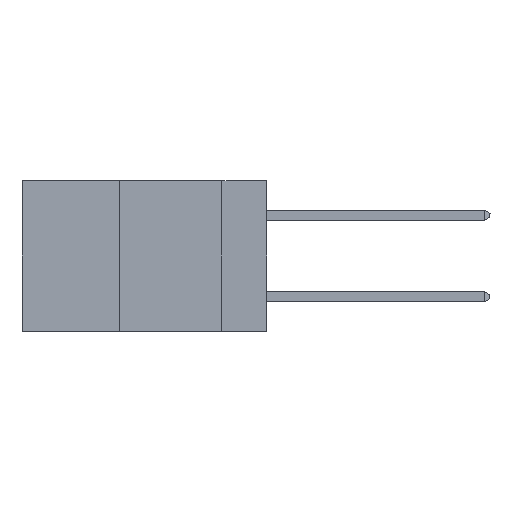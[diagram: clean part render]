
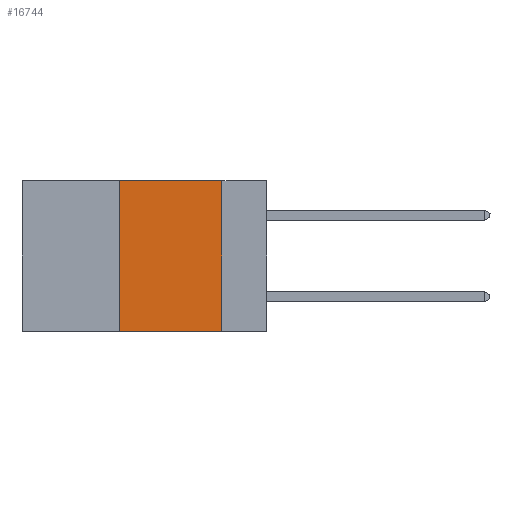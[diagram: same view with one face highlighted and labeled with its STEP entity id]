
A CAD part, left-side view. The second image highlights one B-rep face of the part: STEP entity #16744.
In plain terms, the highlighted planar face has unit normal (-1, 0, 0).
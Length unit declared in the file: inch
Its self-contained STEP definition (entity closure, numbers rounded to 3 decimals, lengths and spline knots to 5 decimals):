
#460 = CARTESIAN_POINT ( 'NONE',  ( 0., 0.36, -0.37 ) ) ;
#677 = EDGE_CURVE ( 'NONE', #7073, #7030, #15146, .T. ) ;
#890 = FACE_OUTER_BOUND ( 'NONE', #3296, .T. ) ;
#1774 = VERTEX_POINT ( 'NONE', #4174 ) ;
#2031 = ORIENTED_EDGE ( 'NONE', *, *, #677, .F. ) ;
#3122 = DIRECTION ( 'NONE',  ( 0., -1., 0. ) ) ;
#3191 = CARTESIAN_POINT ( 'NONE',  ( 0., 0.36, 0. ) ) ;
#3296 = EDGE_LOOP ( 'NONE', ( #5022, #12490, #2031, #5305 ) ) ;
#3569 = EDGE_CURVE ( 'NONE', #7030, #1774, #18235, .T. ) ;
#3662 = AXIS2_PLACEMENT_3D ( 'NONE', #6829, #16704, #9662 ) ;
#3714 = EDGE_CURVE ( 'NONE', #1774, #14645, #5711, .T. ) ;
#4174 = CARTESIAN_POINT ( 'NONE',  ( 0., 0.11, 0. ) ) ;
#5022 = ORIENTED_EDGE ( 'NONE', *, *, #3714, .F. ) ;
#5305 = ORIENTED_EDGE ( 'NONE', *, *, #9707, .T. ) ;
#5711 = LINE ( 'NONE', #13032, #16063 ) ;
#6829 = CARTESIAN_POINT ( 'NONE',  ( 0., 0.6, 0. ) ) ;
#7030 = VERTEX_POINT ( 'NONE', #3191 ) ;
#7073 = VERTEX_POINT ( 'NONE', #460 ) ;
#8883 = VECTOR ( 'NONE', #18135, 39.37008 ) ;
#9662 = DIRECTION ( 'NONE',  ( 0., 0., -1. ) ) ;
#9707 = EDGE_CURVE ( 'NONE', #7073, #14645, #17239, .T. ) ;
#10163 = VECTOR ( 'NONE', #10742, 39.37008 ) ;
#10742 = DIRECTION ( 'NONE',  ( 0., 0., 1. ) ) ;
#11535 = DIRECTION ( 'NONE',  ( 0., 0., -1. ) ) ;
#11597 = CARTESIAN_POINT ( 'NONE',  ( 0., 0.6, -0.37 ) ) ;
#12490 = ORIENTED_EDGE ( 'NONE', *, *, #3569, .F. ) ;
#13032 = CARTESIAN_POINT ( 'NONE',  ( 0., 0.11, 0. ) ) ;
#14175 = CARTESIAN_POINT ( 'NONE',  ( 0., 0.6, 0. ) ) ;
#14645 = VERTEX_POINT ( 'NONE', #16032 ) ;
#15146 = LINE ( 'NONE', #16477, #10163 ) ;
#15226 = VECTOR ( 'NONE', #3122, 39.37008 ) ;
#16032 = CARTESIAN_POINT ( 'NONE',  ( 0., 0.11, -0.37 ) ) ;
#16063 = VECTOR ( 'NONE', #11535, 39.37008 ) ;
#16477 = CARTESIAN_POINT ( 'NONE',  ( 0., 0.36, 0. ) ) ;
#16704 = DIRECTION ( 'NONE',  ( 1., 0., 0. ) ) ;
#16744 = ADVANCED_FACE ( 'NONE', ( #890 ), #18301, .F. ) ;
#17239 = LINE ( 'NONE', #11597, #15226 ) ;
#18135 = DIRECTION ( 'NONE',  ( 0., -1., 0. ) ) ;
#18235 = LINE ( 'NONE', #14175, #8883 ) ;
#18301 = PLANE ( 'NONE',  #3662 ) ;
